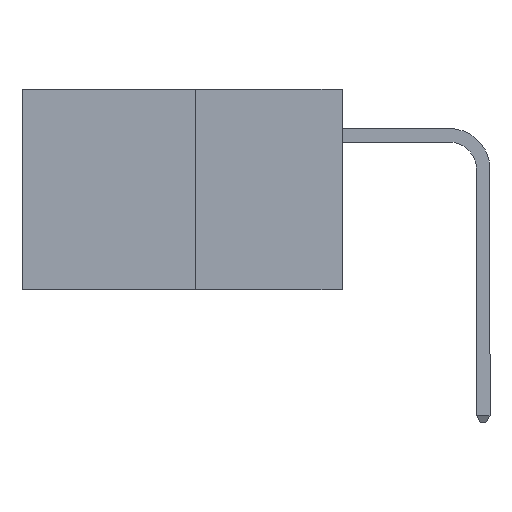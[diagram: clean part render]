
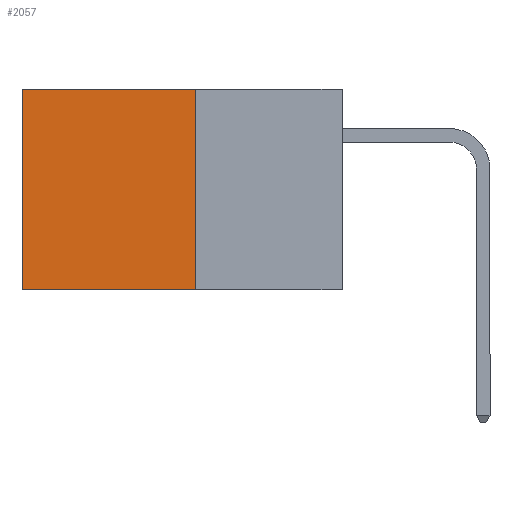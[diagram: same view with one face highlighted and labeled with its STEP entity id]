
A CAD part, left-side view. The second image highlights one B-rep face of the part: STEP entity #2057.
In plain terms, the highlighted planar face has unit normal (-1, 0, 0).
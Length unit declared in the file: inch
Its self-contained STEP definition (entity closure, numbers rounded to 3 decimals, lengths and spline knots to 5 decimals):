
#926 = VECTOR ( 'NONE', #5108, 39.37008 ) ;
#1447 = ORIENTED_EDGE ( 'NONE', *, *, #3158, .F. ) ;
#2057 = ADVANCED_FACE ( 'NONE', ( #4014 ), #21318, .F. ) ;
#2341 = VECTOR ( 'NONE', #16891, 39.37008 ) ;
#2798 = CARTESIAN_POINT ( 'NONE',  ( 0.277, 0.27, 0. ) ) ;
#3028 = CARTESIAN_POINT ( 'NONE',  ( 0.277, 0.59, -0.37 ) ) ;
#3158 = EDGE_CURVE ( 'NONE', #4031, #26013, #24425, .T. ) ;
#4014 = FACE_OUTER_BOUND ( 'NONE', #19786, .T. ) ;
#4031 = VERTEX_POINT ( 'NONE', #2798 ) ;
#5108 = DIRECTION ( 'NONE',  ( 0., 0., -1. ) ) ;
#6405 = VECTOR ( 'NONE', #16207, 39.37008 ) ;
#7216 = ORIENTED_EDGE ( 'NONE', *, *, #12147, .T. ) ;
#8322 = CARTESIAN_POINT ( 'NONE',  ( 0.277, 0.27, -0.37 ) ) ;
#11528 = CARTESIAN_POINT ( 'NONE',  ( 0.277, 0.59, -0.37 ) ) ;
#11803 = LINE ( 'NONE', #3028, #926 ) ;
#11805 = LINE ( 'NONE', #14163, #6405 ) ;
#12147 = EDGE_CURVE ( 'NONE', #4031, #14554, #11805, .T. ) ;
#13408 = CARTESIAN_POINT ( 'NONE',  ( 0.277, 0.27, -0.37 ) ) ;
#13562 = DIRECTION ( 'NONE',  ( 0., 1., 0. ) ) ;
#14163 = CARTESIAN_POINT ( 'NONE',  ( 0.277, 0.27, 0. ) ) ;
#14244 = VERTEX_POINT ( 'NONE', #11528 ) ;
#14554 = VERTEX_POINT ( 'NONE', #16503 ) ;
#15566 = AXIS2_PLACEMENT_3D ( 'NONE', #21175, #22522, #23174 ) ;
#16004 = VECTOR ( 'NONE', #13562, 39.37008 ) ;
#16207 = DIRECTION ( 'NONE',  ( 0., 1., 0. ) ) ;
#16503 = CARTESIAN_POINT ( 'NONE',  ( 0.277, 0.59, 0. ) ) ;
#16891 = DIRECTION ( 'NONE',  ( 0., 0., -1. ) ) ;
#19786 = EDGE_LOOP ( 'NONE', ( #20801, #21475, #1447, #7216 ) ) ;
#20801 = ORIENTED_EDGE ( 'NONE', *, *, #24235, .T. ) ;
#21160 = EDGE_CURVE ( 'NONE', #26013, #14244, #25954, .T. ) ;
#21175 = CARTESIAN_POINT ( 'NONE',  ( 0.277, 0.27, -0.37 ) ) ;
#21318 = PLANE ( 'NONE',  #15566 ) ;
#21475 = ORIENTED_EDGE ( 'NONE', *, *, #21160, .F. ) ;
#22522 = DIRECTION ( 'NONE',  ( 1., 0., 0. ) ) ;
#23174 = DIRECTION ( 'NONE',  ( 0., 0., -1. ) ) ;
#24235 = EDGE_CURVE ( 'NONE', #14554, #14244, #11803, .T. ) ;
#24425 = LINE ( 'NONE', #8322, #2341 ) ;
#25517 = CARTESIAN_POINT ( 'NONE',  ( 0.277, 0.27, -0.37 ) ) ;
#25954 = LINE ( 'NONE', #25517, #16004 ) ;
#26013 = VERTEX_POINT ( 'NONE', #13408 ) ;
